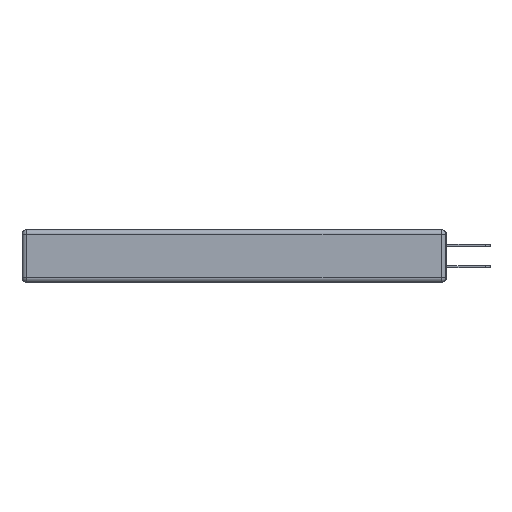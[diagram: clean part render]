
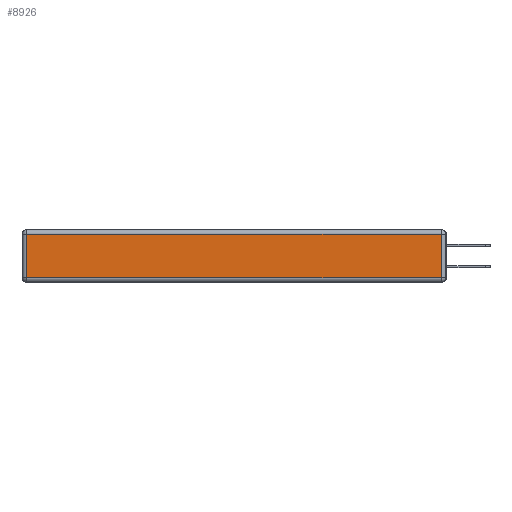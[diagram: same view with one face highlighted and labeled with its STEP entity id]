
A CAD part, left-side view. The second image highlights one B-rep face of the part: STEP entity #8926.
In plain terms, the highlighted planar face has unit normal (-1, 0, 0).
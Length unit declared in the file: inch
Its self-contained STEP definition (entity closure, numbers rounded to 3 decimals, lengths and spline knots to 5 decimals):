
#390 = CARTESIAN_POINT ( 'NONE',  ( 0., 0.03, -0.03 ) ) ;
#1348 = VECTOR ( 'NONE', #5442, 39.37008 ) ;
#1419 = DIRECTION ( 'NONE',  ( 0., 0., -1. ) ) ;
#1594 = CARTESIAN_POINT ( 'NONE',  ( 0., 2.72, -0.343 ) ) ;
#2186 = LINE ( 'NONE', #2561, #26051 ) ;
#2561 = CARTESIAN_POINT ( 'NONE',  ( 0., 2.75, -0.03 ) ) ;
#3373 = AXIS2_PLACEMENT_3D ( 'NONE', #20036, #20226, #9815 ) ;
#4097 = CARTESIAN_POINT ( 'NONE',  ( 0., 0.03, -0.313 ) ) ;
#5442 = DIRECTION ( 'NONE',  ( 0., -1., 0. ) ) ;
#5793 = VERTEX_POINT ( 'NONE', #8620 ) ;
#6188 = EDGE_LOOP ( 'NONE', ( #6511, #15496, #7439, #19812 ) ) ;
#6511 = ORIENTED_EDGE ( 'NONE', *, *, #17449, .T. ) ;
#7439 = ORIENTED_EDGE ( 'NONE', *, *, #26073, .T. ) ;
#7985 = LINE ( 'NONE', #15706, #1348 ) ;
#8620 = CARTESIAN_POINT ( 'NONE',  ( 0., 2.72, -0.03 ) ) ;
#8926 = ADVANCED_FACE ( 'NONE', ( #9523 ), #20323, .T. ) ;
#9523 = FACE_OUTER_BOUND ( 'NONE', #6188, .T. ) ;
#9815 = DIRECTION ( 'NONE',  ( 0., 0., 1. ) ) ;
#10038 = EDGE_CURVE ( 'NONE', #20068, #25735, #13816, .T. ) ;
#10430 = CARTESIAN_POINT ( 'NONE',  ( 0., 0.03, -0.343 ) ) ;
#13816 = LINE ( 'NONE', #10430, #24227 ) ;
#15165 = EDGE_CURVE ( 'NONE', #5793, #26386, #25292, .T. ) ;
#15178 = VECTOR ( 'NONE', #1419, 39.37008 ) ;
#15496 = ORIENTED_EDGE ( 'NONE', *, *, #10038, .T. ) ;
#15706 = CARTESIAN_POINT ( 'NONE',  ( 0., 0., -0.313 ) ) ;
#16354 = CARTESIAN_POINT ( 'NONE',  ( 0., 2.72, -0.313 ) ) ;
#17449 = EDGE_CURVE ( 'NONE', #26386, #20068, #7985, .T. ) ;
#19812 = ORIENTED_EDGE ( 'NONE', *, *, #15165, .T. ) ;
#20036 = CARTESIAN_POINT ( 'NONE',  ( 0., 0., -0.343 ) ) ;
#20068 = VERTEX_POINT ( 'NONE', #4097 ) ;
#20226 = DIRECTION ( 'NONE',  ( -1., 0., 0. ) ) ;
#20323 = PLANE ( 'NONE',  #3373 ) ;
#21487 = DIRECTION ( 'NONE',  ( 0., 1., 0. ) ) ;
#24227 = VECTOR ( 'NONE', #26899, 39.37008 ) ;
#25292 = LINE ( 'NONE', #1594, #15178 ) ;
#25735 = VERTEX_POINT ( 'NONE', #390 ) ;
#26051 = VECTOR ( 'NONE', #21487, 39.37008 ) ;
#26073 = EDGE_CURVE ( 'NONE', #25735, #5793, #2186, .T. ) ;
#26386 = VERTEX_POINT ( 'NONE', #16354 ) ;
#26899 = DIRECTION ( 'NONE',  ( 0., 0., 1. ) ) ;
